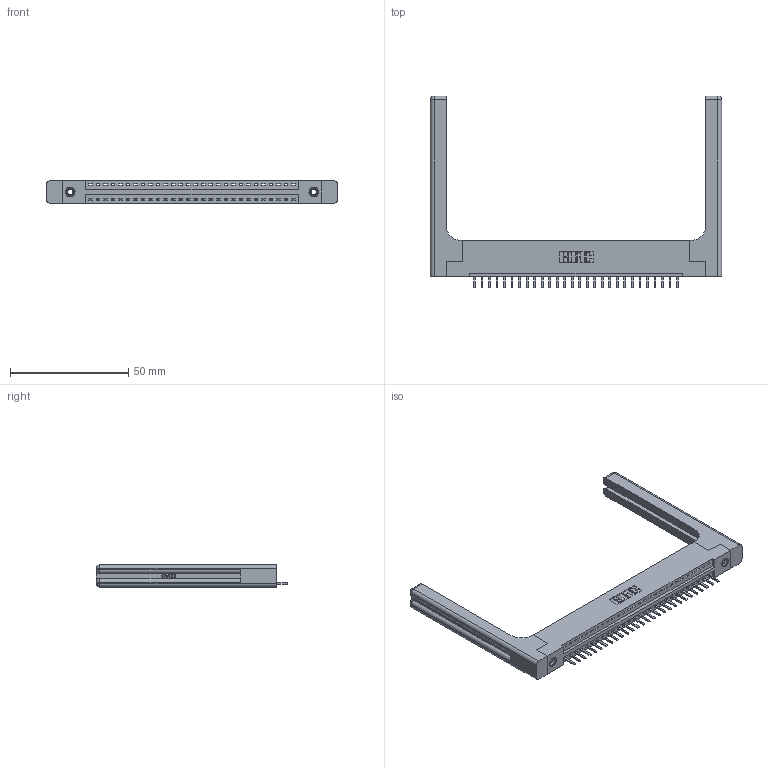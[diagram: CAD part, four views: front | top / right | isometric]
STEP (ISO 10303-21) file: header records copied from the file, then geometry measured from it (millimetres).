
FILE_DESCRIPTION (( 'STEP AP203' ), '1' );
FILE_NAME ('396-028-520-158.STEP', '2019-10-27T08:23:35', ( '' ), ( '' ), 'SwSTEP 2.0', 'SolidWorks 2016', '' );
FILE_SCHEMA (( 'CONFIG_CONTROL_DESIGN' ));
Length unit declared in the file: inch
Products named in the file (5): 346-220-058_345-220-058; 345-292-001_345-293-120; 345-250-001_345-250-001-102; 396-028-520-158; 346 Part_Flush Mounting Lugs - 0.156 Dia-TH
Assembly tree (33 placements, depth 2):
  396-028-520-158
    346 Part_Flush Mounting Lugs - 0.156 Dia-TH
    345-292-001_345-293-120  x28
    345-250-001_345-250-001-102  x2
    346-220-058_345-220-058  x2
Bounding box: 122.96 x 80.98 x 9.4 mm (x, y, z)
Volume: 19111.5 mm3; surface area: 19239.5 mm2
Topology: 33 solids, 33 shells, 2114 faces, 6147 edges, 4002 vertices
Faces by surface type: plane 1400, cylinder 654, bspline 36, cone 12, sphere 8, torus 4
Entity records: 24558 total; most frequent: CARTESIAN_POINT 5205, ORIENTED_EDGE 3952, DIRECTION 3528, EDGE_CURVE 1976, LINE 1636, VECTOR 1636, VERTEX_POINT 1306, AXIS2_PLACEMENT_3D 946
